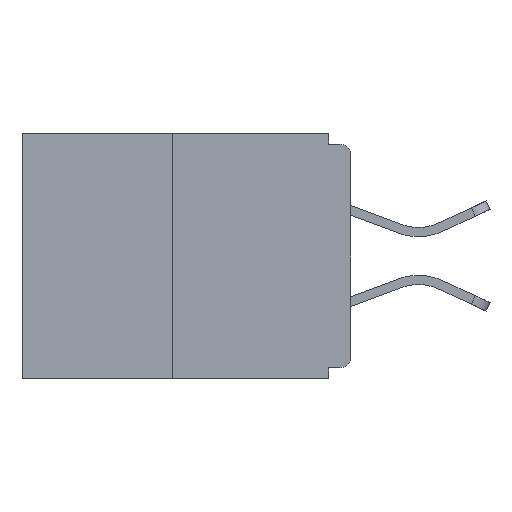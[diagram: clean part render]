
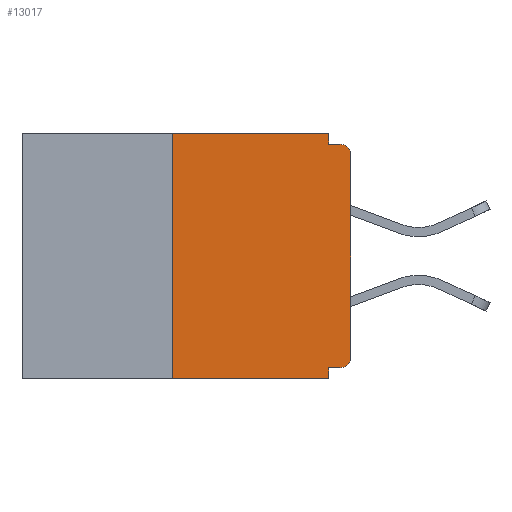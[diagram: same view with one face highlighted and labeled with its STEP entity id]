
A CAD part, left-side view. The second image highlights one B-rep face of the part: STEP entity #13017.
In plain terms, the highlighted planar face has unit normal (-1, 0, 0).
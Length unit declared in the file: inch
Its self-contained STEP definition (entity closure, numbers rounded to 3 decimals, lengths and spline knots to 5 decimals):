
#56 = EDGE_CURVE ( 'NONE', #4232, #15745, #7639, .T. ) ;
#274 = AXIS2_PLACEMENT_3D ( 'NONE', #14606, #5286, #6696 ) ;
#379 = EDGE_CURVE ( 'NONE', #7570, #679, #11328, .T. ) ;
#412 = VERTEX_POINT ( 'NONE', #830 ) ;
#679 = VERTEX_POINT ( 'NONE', #11010 ) ;
#830 = CARTESIAN_POINT ( 'NONE',  ( 0., 0.015, -0.328 ) ) ;
#953 = VERTEX_POINT ( 'NONE', #10287 ) ;
#1009 = DIRECTION ( 'NONE',  ( 0., 0., -1. ) ) ;
#1248 = EDGE_LOOP ( 'NONE', ( #1850, #16389, #5323, #12931, #15688, #8900, #3088, #3532, #5199, #6285 ) ) ;
#1356 = CARTESIAN_POINT ( 'NONE',  ( 0., 0., -0.03 ) ) ;
#1705 = VECTOR ( 'NONE', #13034, 39.37008 ) ;
#1824 = CARTESIAN_POINT ( 'NONE',  ( 0., 0., -0.313 ) ) ;
#1850 = ORIENTED_EDGE ( 'NONE', *, *, #10756, .F. ) ;
#2384 = CARTESIAN_POINT ( 'NONE',  ( 0., 0.46, 0. ) ) ;
#2636 = PLANE ( 'NONE',  #18187 ) ;
#2660 = VERTEX_POINT ( 'NONE', #5687 ) ;
#2789 = EDGE_CURVE ( 'NONE', #8143, #953, #6797, .T. ) ;
#2920 = DIRECTION ( 'NONE',  ( 0., 0., 1. ) ) ;
#3088 = ORIENTED_EDGE ( 'NONE', *, *, #56, .T. ) ;
#3336 = LINE ( 'NONE', #14467, #1705 ) ;
#3532 = ORIENTED_EDGE ( 'NONE', *, *, #7536, .T. ) ;
#3869 = DIRECTION ( 'NONE',  ( 0., 0., -1. ) ) ;
#4232 = VERTEX_POINT ( 'NONE', #1824 ) ;
#4365 = CIRCLE ( 'NONE', #274, 0.015 ) ;
#4461 = EDGE_CURVE ( 'NONE', #7570, #16551, #8498, .T. ) ;
#5199 = ORIENTED_EDGE ( 'NONE', *, *, #18454, .F. ) ;
#5286 = DIRECTION ( 'NONE',  ( -1., 0., 0. ) ) ;
#5323 = ORIENTED_EDGE ( 'NONE', *, *, #4461, .T. ) ;
#5687 = CARTESIAN_POINT ( 'NONE',  ( 0., 0.031, -0.328 ) ) ;
#5832 = CIRCLE ( 'NONE', #13375, 0.015 ) ;
#6184 = DIRECTION ( 'NONE',  ( 0., 1., 0. ) ) ;
#6285 = ORIENTED_EDGE ( 'NONE', *, *, #2789, .F. ) ;
#6646 = LINE ( 'NONE', #15092, #12478 ) ;
#6696 = DIRECTION ( 'NONE',  ( 0., 0., -1. ) ) ;
#6797 = LINE ( 'NONE', #18940, #9838 ) ;
#6979 = EDGE_CURVE ( 'NONE', #2660, #16551, #3336, .T. ) ;
#7331 = CARTESIAN_POINT ( 'NONE',  ( 0., 0., 0. ) ) ;
#7363 = CARTESIAN_POINT ( 'NONE',  ( 0., 0.46, -0.343 ) ) ;
#7391 = VECTOR ( 'NONE', #2920, 39.37008 ) ;
#7536 = EDGE_CURVE ( 'NONE', #15745, #12170, #5832, .T. ) ;
#7570 = VERTEX_POINT ( 'NONE', #9912 ) ;
#7615 = DIRECTION ( 'NONE',  ( 0., -1., 0. ) ) ;
#7639 = LINE ( 'NONE', #7331, #14383 ) ;
#7836 = CARTESIAN_POINT ( 'NONE',  ( 0., 0., -0.015 ) ) ;
#8084 = LINE ( 'NONE', #12109, #17377 ) ;
#8143 = VERTEX_POINT ( 'NONE', #9437 ) ;
#8356 = DIRECTION ( 'NONE',  ( -1., 0., 0. ) ) ;
#8498 = LINE ( 'NONE', #7363, #11276 ) ;
#8671 = VECTOR ( 'NONE', #10743, 39.37008 ) ;
#8900 = ORIENTED_EDGE ( 'NONE', *, *, #10969, .T. ) ;
#9437 = CARTESIAN_POINT ( 'NONE',  ( 0., 0.031, 0. ) ) ;
#9838 = VECTOR ( 'NONE', #10106, 39.37008 ) ;
#9912 = CARTESIAN_POINT ( 'NONE',  ( 0., 0.25, -0.343 ) ) ;
#10106 = DIRECTION ( 'NONE',  ( 0., 0., -1. ) ) ;
#10287 = CARTESIAN_POINT ( 'NONE',  ( 0., 0.031, -0.015 ) ) ;
#10301 = DIRECTION ( 'NONE',  ( 0., 0., 1. ) ) ;
#10454 = CARTESIAN_POINT ( 'NONE',  ( 0., 0.25, 0. ) ) ;
#10479 = CARTESIAN_POINT ( 'NONE',  ( 0., 0.015, -0.015 ) ) ;
#10743 = DIRECTION ( 'NONE',  ( 0., -1., 0. ) ) ;
#10756 = EDGE_CURVE ( 'NONE', #679, #8143, #8084, .T. ) ;
#10969 = EDGE_CURVE ( 'NONE', #412, #4232, #4365, .T. ) ;
#11010 = CARTESIAN_POINT ( 'NONE',  ( 0., 0.25, 0. ) ) ;
#11276 = VECTOR ( 'NONE', #17747, 39.37008 ) ;
#11328 = LINE ( 'NONE', #10454, #7391 ) ;
#11332 = CARTESIAN_POINT ( 'NONE',  ( 0., 0.015, -0.03 ) ) ;
#12109 = CARTESIAN_POINT ( 'NONE',  ( 0., 0.46, 0. ) ) ;
#12170 = VERTEX_POINT ( 'NONE', #10479 ) ;
#12478 = VECTOR ( 'NONE', #6184, 39.37008 ) ;
#12931 = ORIENTED_EDGE ( 'NONE', *, *, #6979, .F. ) ;
#13017 = ADVANCED_FACE ( 'NONE', ( #17327 ), #2636, .F. ) ;
#13034 = DIRECTION ( 'NONE',  ( 0., 0., -1. ) ) ;
#13341 = CARTESIAN_POINT ( 'NONE',  ( 0., 0.031, -0.343 ) ) ;
#13375 = AXIS2_PLACEMENT_3D ( 'NONE', #11332, #8356, #3869 ) ;
#14383 = VECTOR ( 'NONE', #10301, 39.37008 ) ;
#14467 = CARTESIAN_POINT ( 'NONE',  ( 0., 0.031, -0.343 ) ) ;
#14606 = CARTESIAN_POINT ( 'NONE',  ( 0., 0.015, -0.313 ) ) ;
#15092 = CARTESIAN_POINT ( 'NONE',  ( 0., 0., -0.328 ) ) ;
#15688 = ORIENTED_EDGE ( 'NONE', *, *, #17001, .F. ) ;
#15745 = VERTEX_POINT ( 'NONE', #1356 ) ;
#16389 = ORIENTED_EDGE ( 'NONE', *, *, #379, .F. ) ;
#16551 = VERTEX_POINT ( 'NONE', #13341 ) ;
#17001 = EDGE_CURVE ( 'NONE', #412, #2660, #6646, .T. ) ;
#17211 = DIRECTION ( 'NONE',  ( 1., 0., 0. ) ) ;
#17327 = FACE_OUTER_BOUND ( 'NONE', #1248, .T. ) ;
#17377 = VECTOR ( 'NONE', #7615, 39.37008 ) ;
#17747 = DIRECTION ( 'NONE',  ( 0., -1., 0. ) ) ;
#17975 = LINE ( 'NONE', #7836, #8671 ) ;
#18187 = AXIS2_PLACEMENT_3D ( 'NONE', #2384, #17211, #1009 ) ;
#18454 = EDGE_CURVE ( 'NONE', #953, #12170, #17975, .T. ) ;
#18940 = CARTESIAN_POINT ( 'NONE',  ( 0., 0.031, 0. ) ) ;
